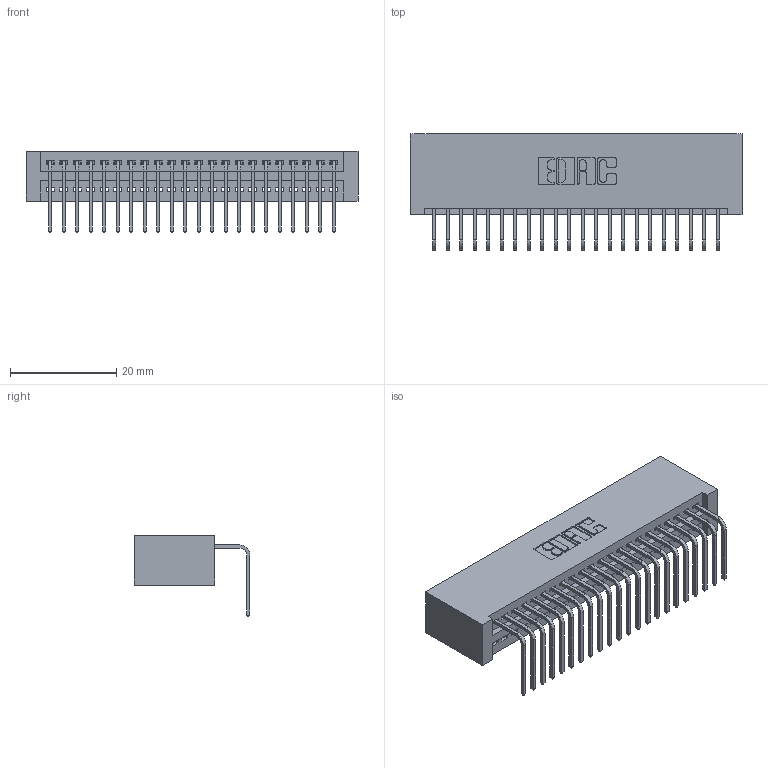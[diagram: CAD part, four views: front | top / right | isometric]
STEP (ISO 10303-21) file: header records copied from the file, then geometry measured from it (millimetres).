
FILE_DESCRIPTION (( 'STEP AP203' ), '1' );
FILE_NAME ('395-022-558-101.STEP', '2019-10-11T04:24:15', ( '' ), ( '' ), 'SwSTEP 2.0', 'SolidWorks 2016', '' );
FILE_SCHEMA (( 'CONFIG_CONTROL_DESIGN' ));
Length unit declared in the file: inch
Products named in the file (3): 345 Part_No Mounting Lugs; 345-292-001_558 Tail - 2; 395-022-558-101
Assembly tree (23 placements, depth 2):
  395-022-558-101
    345 Part_No Mounting Lugs
    345-292-001_558 Tail - 2  x22
Bounding box: 62.48 x 21.83 x 15.37 mm (x, y, z)
Volume: 6428.6 mm3; surface area: 8892.1 mm2
Topology: 23 solids, 23 shells, 1438 faces, 4321 edges, 2850 vertices
Faces by surface type: plane 1000, cylinder 438
Entity records: 19057 total; most frequent: CARTESIAN_POINT 3310, ORIENTED_EDGE 3266, DIRECTION 2913, EDGE_CURVE 1633, VECTOR 1421, LINE 1421, VERTEX_POINT 1086, AXIS2_PLACEMENT_3D 746
